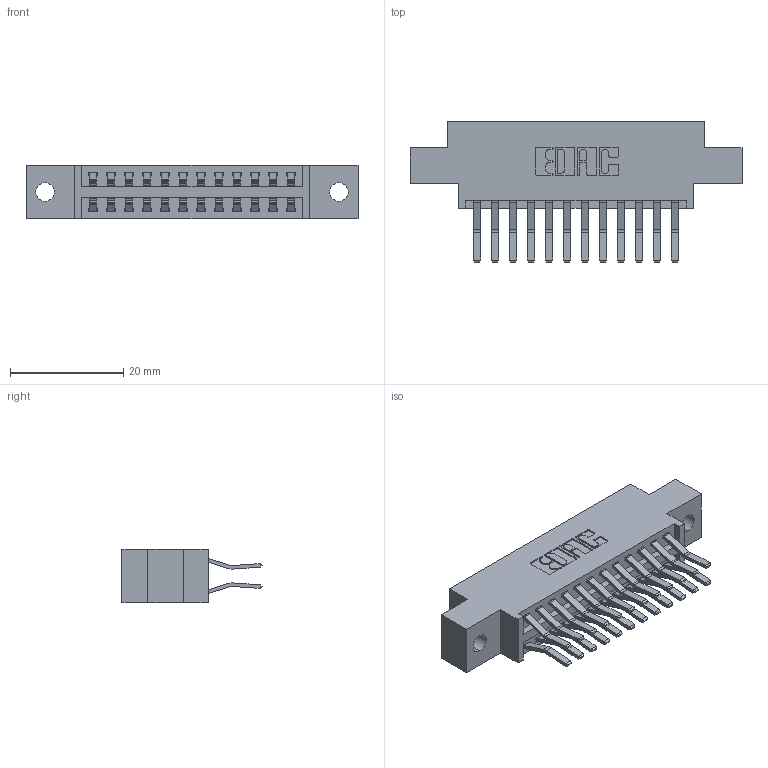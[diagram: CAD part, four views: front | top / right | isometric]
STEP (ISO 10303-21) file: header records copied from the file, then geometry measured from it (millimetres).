
FILE_DESCRIPTION (( 'STEP AP203' ), '1' );
FILE_NAME ('346-024-560-802.STEP', '2022-05-19T00:42:54', ( '' ), ( '' ), 'SwSTEP 2.0', 'SolidWorks 2020', '' );
FILE_SCHEMA (( 'CONFIG_CONTROL_DESIGN' ));
Length unit declared in the file: inch
Products named in the file (3): 346 Part_0.170 Offset - 0.128 Dia; 345-292-001_560 Tail; 346-024-560-802
Assembly tree (25 placements, depth 2):
  346-024-560-802
    346 Part_0.170 Offset - 0.128 Dia
    345-292-001_560 Tail  x24
Bounding box: 58.67 x 24.78 x 9.4 mm (x, y, z)
Volume: 5454.5 mm3; surface area: 7356.1 mm2
Topology: 25 solids, 25 shells, 1422 faces, 4205 edges, 2770 vertices
Faces by surface type: plane 920, cylinder 502
Entity records: 12093 total; most frequent: CARTESIAN_POINT 2036, ORIENTED_EDGE 1970, DIRECTION 1849, EDGE_CURVE 985, VECTOR 801, LINE 801, VERTEX_POINT 654, AXIS2_PLACEMENT_3D 524
